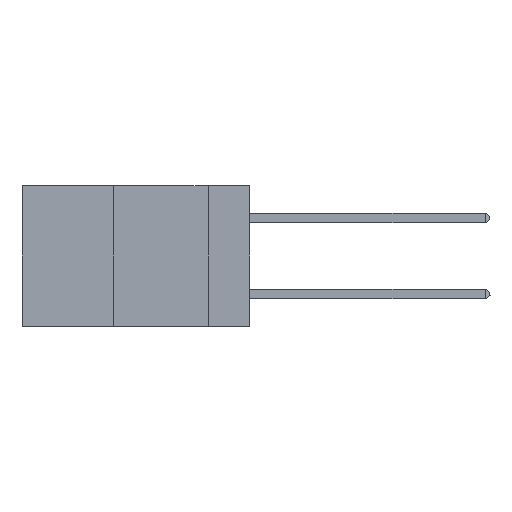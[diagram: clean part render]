
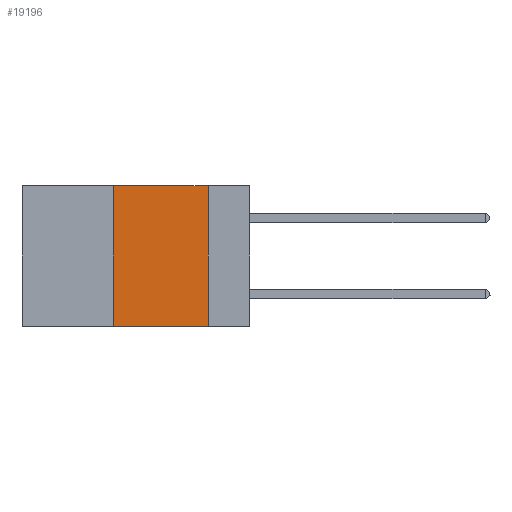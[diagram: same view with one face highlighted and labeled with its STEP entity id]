
A CAD part, left-side view. The second image highlights one B-rep face of the part: STEP entity #19196.
In plain terms, the highlighted planar face has unit normal (-1, 0, 0).
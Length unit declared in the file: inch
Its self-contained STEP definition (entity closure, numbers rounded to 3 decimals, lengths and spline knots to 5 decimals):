
#964 = DIRECTION ( 'NONE',  ( 0., -1., 0. ) ) ;
#1300 = CARTESIAN_POINT ( 'NONE',  ( 0., 0.6, -0.37 ) ) ;
#2812 = EDGE_CURVE ( 'NONE', #11351, #19330, #4541, .T. ) ;
#2925 = PLANE ( 'NONE',  #23167 ) ;
#4007 = VERTEX_POINT ( 'NONE', #6786 ) ;
#4541 = LINE ( 'NONE', #27456, #14708 ) ;
#4595 = LINE ( 'NONE', #21164, #25731 ) ;
#6786 = CARTESIAN_POINT ( 'NONE',  ( 0., 0.36, 0. ) ) ;
#7153 = LINE ( 'NONE', #1300, #10804 ) ;
#7491 = FACE_OUTER_BOUND ( 'NONE', #28453, .T. ) ;
#8087 = DIRECTION ( 'NONE',  ( 0., 0., -1. ) ) ;
#8604 = CARTESIAN_POINT ( 'NONE',  ( 0., 0.11, 0. ) ) ;
#10379 = CARTESIAN_POINT ( 'NONE',  ( 0., 0.6, 0. ) ) ;
#10804 = VECTOR ( 'NONE', #964, 39.37008 ) ;
#11351 = VERTEX_POINT ( 'NONE', #8604 ) ;
#12400 = EDGE_CURVE ( 'NONE', #28163, #19330, #7153, .T. ) ;
#13641 = EDGE_CURVE ( 'NONE', #4007, #11351, #4595, .T. ) ;
#14708 = VECTOR ( 'NONE', #30102, 39.37008 ) ;
#16629 = LINE ( 'NONE', #28461, #20692 ) ;
#17245 = CARTESIAN_POINT ( 'NONE',  ( 0., 0.11, -0.37 ) ) ;
#19196 = ADVANCED_FACE ( 'NONE', ( #7491 ), #2925, .F. ) ;
#19330 = VERTEX_POINT ( 'NONE', #17245 ) ;
#20692 = VECTOR ( 'NONE', #25942, 39.37008 ) ;
#21033 = DIRECTION ( 'NONE',  ( 1., 0., 0. ) ) ;
#21164 = CARTESIAN_POINT ( 'NONE',  ( 0., 0.6, 0. ) ) ;
#22191 = EDGE_CURVE ( 'NONE', #28163, #4007, #16629, .T. ) ;
#23167 = AXIS2_PLACEMENT_3D ( 'NONE', #10379, #21033, #8087 ) ;
#24824 = CARTESIAN_POINT ( 'NONE',  ( 0., 0.36, -0.37 ) ) ;
#25204 = ORIENTED_EDGE ( 'NONE', *, *, #13641, .F. ) ;
#25439 = ORIENTED_EDGE ( 'NONE', *, *, #2812, .F. ) ;
#25731 = VECTOR ( 'NONE', #26382, 39.37008 ) ;
#25942 = DIRECTION ( 'NONE',  ( 0., 0., 1. ) ) ;
#26382 = DIRECTION ( 'NONE',  ( 0., -1., 0. ) ) ;
#27456 = CARTESIAN_POINT ( 'NONE',  ( 0., 0.11, 0. ) ) ;
#28163 = VERTEX_POINT ( 'NONE', #24824 ) ;
#28453 = EDGE_LOOP ( 'NONE', ( #25439, #25204, #32153, #30538 ) ) ;
#28461 = CARTESIAN_POINT ( 'NONE',  ( 0., 0.36, 0. ) ) ;
#30102 = DIRECTION ( 'NONE',  ( 0., 0., -1. ) ) ;
#30538 = ORIENTED_EDGE ( 'NONE', *, *, #12400, .T. ) ;
#32153 = ORIENTED_EDGE ( 'NONE', *, *, #22191, .F. ) ;
